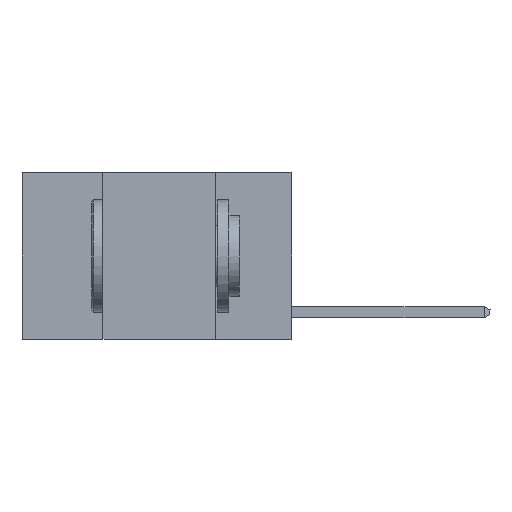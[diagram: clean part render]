
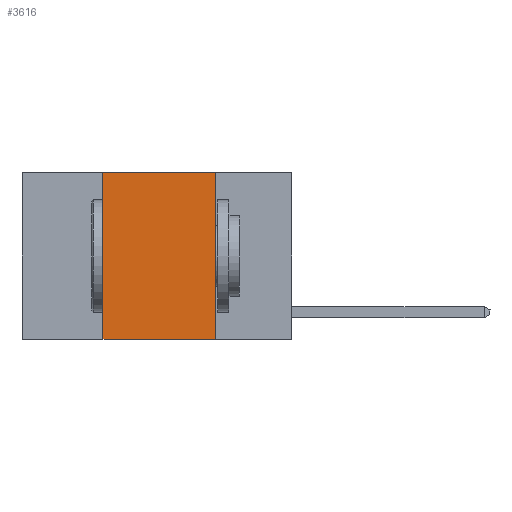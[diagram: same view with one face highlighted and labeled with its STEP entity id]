
A CAD part, left-side view. The second image highlights one B-rep face of the part: STEP entity #3616.
In plain terms, the highlighted planar face has unit normal (-1, 0, 0).
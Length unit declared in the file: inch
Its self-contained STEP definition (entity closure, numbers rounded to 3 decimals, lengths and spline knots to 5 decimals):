
#298 = CARTESIAN_POINT ( 'NONE',  ( 0., 0.42, 0. ) ) ;
#568 = FACE_OUTER_BOUND ( 'NONE', #5679, .T. ) ;
#888 = DIRECTION ( 'NONE',  ( 0., 0., -1. ) ) ;
#946 = DIRECTION ( 'NONE',  ( 1., 0., 0. ) ) ;
#1012 = PLANE ( 'NONE',  #1029 ) ;
#1029 = AXIS2_PLACEMENT_3D ( 'NONE', #1816, #946, #888 ) ;
#1093 = VERTEX_POINT ( 'NONE', #7981 ) ;
#1816 = CARTESIAN_POINT ( 'NONE',  ( 0., 0.6, 0. ) ) ;
#1991 = VECTOR ( 'NONE', #4547, 39.37008 ) ;
#2046 = LINE ( 'NONE', #4180, #1991 ) ;
#2906 = VECTOR ( 'NONE', #4882, 39.37008 ) ;
#3361 = LINE ( 'NONE', #4853, #7218 ) ;
#3616 = ADVANCED_FACE ( 'NONE', ( #568 ), #1012, .F. ) ;
#4019 = CARTESIAN_POINT ( 'NONE',  ( 0., 0.6, -0.37 ) ) ;
#4180 = CARTESIAN_POINT ( 'NONE',  ( 0., 0.6, 0. ) ) ;
#4547 = DIRECTION ( 'NONE',  ( 0., -1., 0. ) ) ;
#4610 = DIRECTION ( 'NONE',  ( 0., -1., 0. ) ) ;
#4755 = DIRECTION ( 'NONE',  ( 0., 0., 1. ) ) ;
#4834 = EDGE_CURVE ( 'NONE', #5526, #8902, #2046, .T. ) ;
#4853 = CARTESIAN_POINT ( 'NONE',  ( 0., 0.42, 0. ) ) ;
#4882 = DIRECTION ( 'NONE',  ( 0., 0., -1. ) ) ;
#4972 = CARTESIAN_POINT ( 'NONE',  ( 0., 0.17, 0. ) ) ;
#5350 = EDGE_CURVE ( 'NONE', #8902, #1093, #8725, .T. ) ;
#5351 = EDGE_CURVE ( 'NONE', #8408, #5526, #3361, .T. ) ;
#5368 = EDGE_CURVE ( 'NONE', #8408, #1093, #7080, .T. ) ;
#5526 = VERTEX_POINT ( 'NONE', #298 ) ;
#5679 = EDGE_LOOP ( 'NONE', ( #5834, #6064, #5794, #5821 ) ) ;
#5794 = ORIENTED_EDGE ( 'NONE', *, *, #5351, .F. ) ;
#5821 = ORIENTED_EDGE ( 'NONE', *, *, #5368, .T. ) ;
#5834 = ORIENTED_EDGE ( 'NONE', *, *, #5350, .F. ) ;
#6064 = ORIENTED_EDGE ( 'NONE', *, *, #4834, .F. ) ;
#6864 = CARTESIAN_POINT ( 'NONE',  ( 0., 0.17, 0. ) ) ;
#7080 = LINE ( 'NONE', #4019, #8890 ) ;
#7218 = VECTOR ( 'NONE', #4755, 39.37008 ) ;
#7455 = CARTESIAN_POINT ( 'NONE',  ( 0., 0.42, -0.37 ) ) ;
#7981 = CARTESIAN_POINT ( 'NONE',  ( 0., 0.17, -0.37 ) ) ;
#8408 = VERTEX_POINT ( 'NONE', #7455 ) ;
#8725 = LINE ( 'NONE', #4972, #2906 ) ;
#8890 = VECTOR ( 'NONE', #4610, 39.37008 ) ;
#8902 = VERTEX_POINT ( 'NONE', #6864 ) ;
